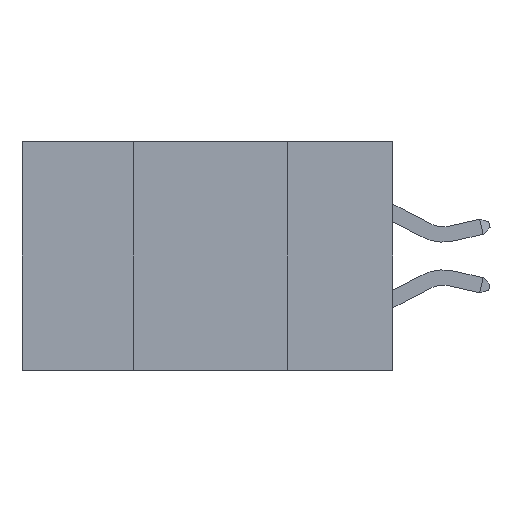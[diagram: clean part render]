
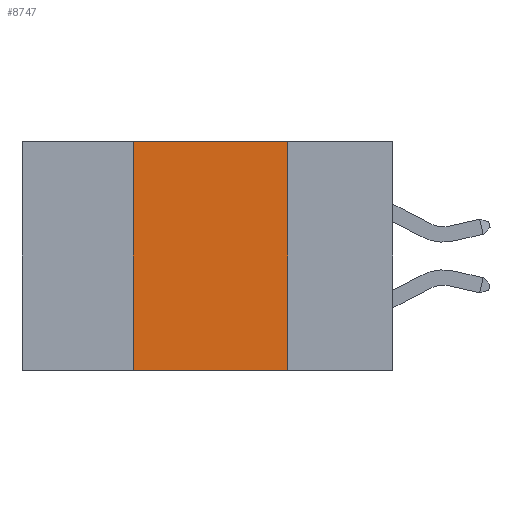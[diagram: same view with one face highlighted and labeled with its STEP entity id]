
A CAD part, left-side view. The second image highlights one B-rep face of the part: STEP entity #8747.
In plain terms, the highlighted planar face has unit normal (-1, 0, 0).
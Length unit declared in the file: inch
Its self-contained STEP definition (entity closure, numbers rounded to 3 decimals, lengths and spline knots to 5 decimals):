
#84 = EDGE_CURVE ( 'NONE', #22730, #14619, #8096, .T. ) ;
#760 = CARTESIAN_POINT ( 'NONE',  ( 0., 0.6, 0. ) ) ;
#1620 = CARTESIAN_POINT ( 'NONE',  ( 0., 0.42, -0.37 ) ) ;
#2338 = DIRECTION ( 'NONE',  ( 0., 0., -1. ) ) ;
#2956 = DIRECTION ( 'NONE',  ( 0., -1., 0. ) ) ;
#4363 = PLANE ( 'NONE',  #13858 ) ;
#5583 = EDGE_CURVE ( 'NONE', #17652, #22730, #17530, .T. ) ;
#5720 = VERTEX_POINT ( 'NONE', #7156 ) ;
#6050 = CARTESIAN_POINT ( 'NONE',  ( 0., 0.17, 0. ) ) ;
#7156 = CARTESIAN_POINT ( 'NONE',  ( 0., 0.17, -0.37 ) ) ;
#7956 = ORIENTED_EDGE ( 'NONE', *, *, #13081, .F. ) ;
#8096 = LINE ( 'NONE', #22850, #13482 ) ;
#8102 = DIRECTION ( 'NONE',  ( 1., 0., 0. ) ) ;
#8747 = ADVANCED_FACE ( 'NONE', ( #20470 ), #4363, .F. ) ;
#9095 = CARTESIAN_POINT ( 'NONE',  ( 0., 0.17, 0. ) ) ;
#9749 = ORIENTED_EDGE ( 'NONE', *, *, #84, .F. ) ;
#10005 = DIRECTION ( 'NONE',  ( 0., -1., 0. ) ) ;
#10353 = LINE ( 'NONE', #6050, #11764 ) ;
#10559 = CARTESIAN_POINT ( 'NONE',  ( 0., 0.42, 0. ) ) ;
#10726 = LINE ( 'NONE', #20920, #11851 ) ;
#11764 = VECTOR ( 'NONE', #2338, 39.37008 ) ;
#11851 = VECTOR ( 'NONE', #10005, 39.37008 ) ;
#11875 = DIRECTION ( 'NONE',  ( 0., 0., -1. ) ) ;
#12357 = CARTESIAN_POINT ( 'NONE',  ( 0., 0.42, 0. ) ) ;
#12889 = EDGE_LOOP ( 'NONE', ( #7956, #9749, #14337, #18297 ) ) ;
#13081 = EDGE_CURVE ( 'NONE', #14619, #5720, #10353, .T. ) ;
#13482 = VECTOR ( 'NONE', #2956, 39.37008 ) ;
#13858 = AXIS2_PLACEMENT_3D ( 'NONE', #760, #8102, #11875 ) ;
#14337 = ORIENTED_EDGE ( 'NONE', *, *, #5583, .F. ) ;
#14619 = VERTEX_POINT ( 'NONE', #9095 ) ;
#16725 = EDGE_CURVE ( 'NONE', #17652, #5720, #10726, .T. ) ;
#17530 = LINE ( 'NONE', #12357, #21256 ) ;
#17643 = DIRECTION ( 'NONE',  ( 0., 0., 1. ) ) ;
#17652 = VERTEX_POINT ( 'NONE', #1620 ) ;
#18297 = ORIENTED_EDGE ( 'NONE', *, *, #16725, .T. ) ;
#20470 = FACE_OUTER_BOUND ( 'NONE', #12889, .T. ) ;
#20920 = CARTESIAN_POINT ( 'NONE',  ( 0., 0.6, -0.37 ) ) ;
#21256 = VECTOR ( 'NONE', #17643, 39.37008 ) ;
#22730 = VERTEX_POINT ( 'NONE', #10559 ) ;
#22850 = CARTESIAN_POINT ( 'NONE',  ( 0., 0.6, 0. ) ) ;
